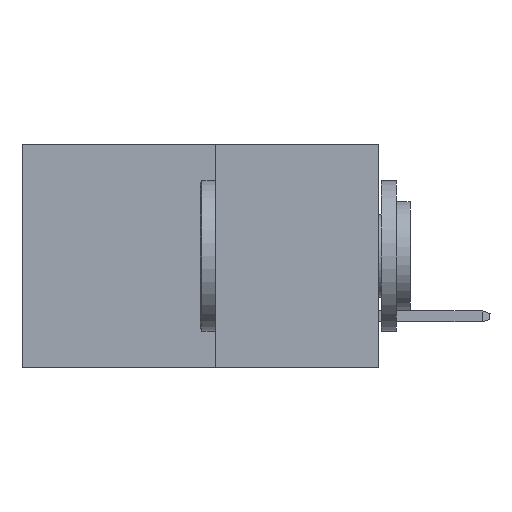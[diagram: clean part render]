
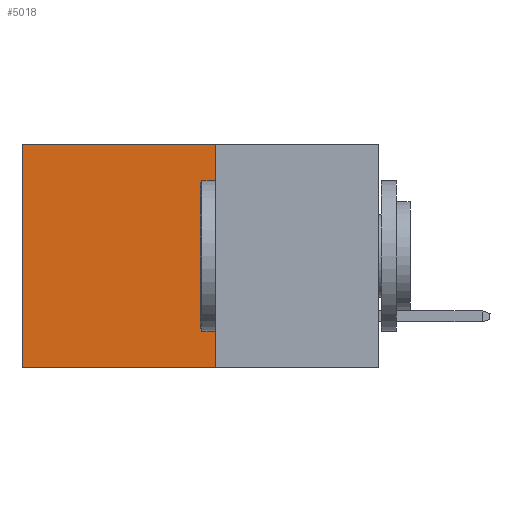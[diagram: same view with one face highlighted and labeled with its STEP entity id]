
A CAD part, left-side view. The second image highlights one B-rep face of the part: STEP entity #5018.
In plain terms, the highlighted planar face has unit normal (-1, 0, 0).
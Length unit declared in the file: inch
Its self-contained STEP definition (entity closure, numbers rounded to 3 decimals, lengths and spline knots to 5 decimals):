
#898 = CARTESIAN_POINT ( 'NONE',  ( 0.277, 0.27, -0.37 ) ) ;
#912 = CARTESIAN_POINT ( 'NONE',  ( 0.277, 0.27, -0.37 ) ) ;
#989 = LINE ( 'NONE', #5486, #3045 ) ;
#1434 = LINE ( 'NONE', #7727, #3713 ) ;
#2332 = EDGE_CURVE ( 'NONE', #7592, #7693, #3207, .T. ) ;
#3045 = VECTOR ( 'NONE', #7165, 39.37008 ) ;
#3207 = LINE ( 'NONE', #898, #6899 ) ;
#3342 = ORIENTED_EDGE ( 'NONE', *, *, #3694, .T. ) ;
#3630 = AXIS2_PLACEMENT_3D ( 'NONE', #8069, #7748, #7733 ) ;
#3694 = EDGE_CURVE ( 'NONE', #4482, #9389, #989, .T. ) ;
#3713 = VECTOR ( 'NONE', #7939, 39.37008 ) ;
#4141 = FACE_OUTER_BOUND ( 'NONE', #6905, .T. ) ;
#4235 = EDGE_CURVE ( 'NONE', #7693, #9389, #1434, .T. ) ;
#4482 = VERTEX_POINT ( 'NONE', #5341 ) ;
#5018 = ADVANCED_FACE ( 'NONE', ( #4141 ), #8155, .F. ) ;
#5041 = DIRECTION ( 'NONE',  ( 0., 1., 0. ) ) ;
#5341 = CARTESIAN_POINT ( 'NONE',  ( 0.277, 0.59, 0. ) ) ;
#5457 = ORIENTED_EDGE ( 'NONE', *, *, #4235, .F. ) ;
#5486 = CARTESIAN_POINT ( 'NONE',  ( 0.277, 0.59, -0.37 ) ) ;
#5929 = VECTOR ( 'NONE', #5041, 39.37008 ) ;
#6016 = CARTESIAN_POINT ( 'NONE',  ( 0.277, 0.59, -0.37 ) ) ;
#6090 = DIRECTION ( 'NONE',  ( 0., 0., -1. ) ) ;
#6899 = VECTOR ( 'NONE', #6090, 39.37008 ) ;
#6905 = EDGE_LOOP ( 'NONE', ( #3342, #5457, #7199, #8773 ) ) ;
#7165 = DIRECTION ( 'NONE',  ( 0., 0., -1. ) ) ;
#7199 = ORIENTED_EDGE ( 'NONE', *, *, #2332, .F. ) ;
#7585 = EDGE_CURVE ( 'NONE', #7592, #4482, #7619, .T. ) ;
#7592 = VERTEX_POINT ( 'NONE', #8188 ) ;
#7594 = CARTESIAN_POINT ( 'NONE',  ( 0.277, 0.27, 0. ) ) ;
#7619 = LINE ( 'NONE', #7594, #5929 ) ;
#7693 = VERTEX_POINT ( 'NONE', #912 ) ;
#7727 = CARTESIAN_POINT ( 'NONE',  ( 0.277, 0.27, -0.37 ) ) ;
#7733 = DIRECTION ( 'NONE',  ( 0., 0., -1. ) ) ;
#7748 = DIRECTION ( 'NONE',  ( 1., 0., 0. ) ) ;
#7939 = DIRECTION ( 'NONE',  ( 0., 1., 0. ) ) ;
#8069 = CARTESIAN_POINT ( 'NONE',  ( 0.277, 0.27, -0.37 ) ) ;
#8155 = PLANE ( 'NONE',  #3630 ) ;
#8188 = CARTESIAN_POINT ( 'NONE',  ( 0.277, 0.27, 0. ) ) ;
#8773 = ORIENTED_EDGE ( 'NONE', *, *, #7585, .T. ) ;
#9389 = VERTEX_POINT ( 'NONE', #6016 ) ;
